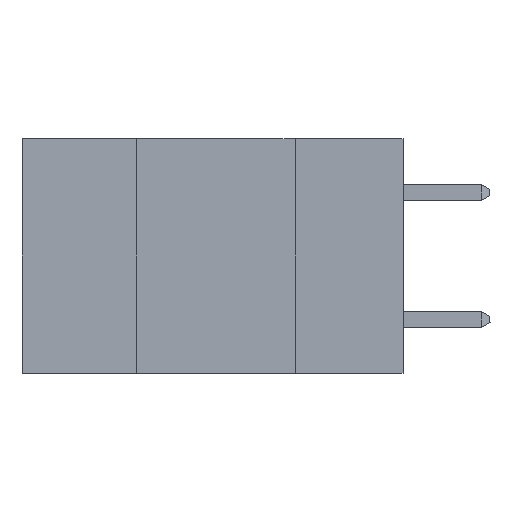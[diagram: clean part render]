
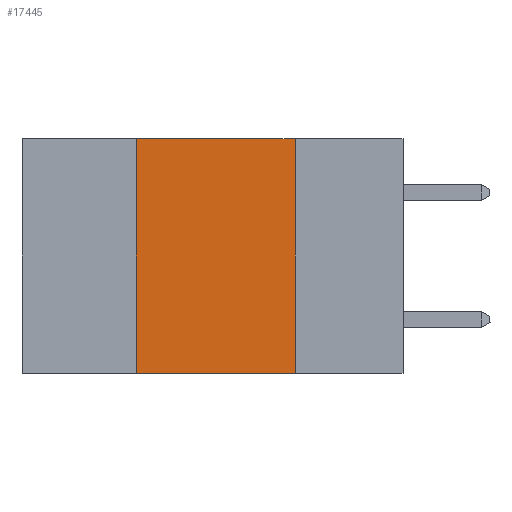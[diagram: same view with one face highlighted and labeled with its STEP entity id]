
A CAD part, left-side view. The second image highlights one B-rep face of the part: STEP entity #17445.
In plain terms, the highlighted planar face has unit normal (-1, 0, 0).
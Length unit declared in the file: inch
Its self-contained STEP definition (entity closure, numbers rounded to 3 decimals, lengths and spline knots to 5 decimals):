
#869 = EDGE_CURVE ( 'NONE', #5063, #23213, #18012, .T. ) ;
#1693 = PLANE ( 'NONE',  #20402 ) ;
#1990 = VERTEX_POINT ( 'NONE', #6628 ) ;
#2086 = CARTESIAN_POINT ( 'NONE',  ( 0., 0.17, 0. ) ) ;
#3601 = ORIENTED_EDGE ( 'NONE', *, *, #27813, .T. ) ;
#4275 = EDGE_CURVE ( 'NONE', #23213, #1990, #21564, .T. ) ;
#5063 = VERTEX_POINT ( 'NONE', #20361 ) ;
#6628 = CARTESIAN_POINT ( 'NONE',  ( 0., 0.17, 0. ) ) ;
#7242 = CARTESIAN_POINT ( 'NONE',  ( 0., 0.6, -0.37 ) ) ;
#7342 = DIRECTION ( 'NONE',  ( 0., -1., 0. ) ) ;
#7933 = EDGE_CURVE ( 'NONE', #1990, #22974, #9952, .T. ) ;
#8249 = FACE_OUTER_BOUND ( 'NONE', #17462, .T. ) ;
#9952 = LINE ( 'NONE', #2086, #22491 ) ;
#10127 = DIRECTION ( 'NONE',  ( 0., -1., 0. ) ) ;
#10980 = VECTOR ( 'NONE', #19770, 39.37008 ) ;
#11311 = CARTESIAN_POINT ( 'NONE',  ( 0., 0.6, 0. ) ) ;
#12467 = CARTESIAN_POINT ( 'NONE',  ( 0., 0.17, -0.37 ) ) ;
#16337 = ORIENTED_EDGE ( 'NONE', *, *, #869, .F. ) ;
#17445 = ADVANCED_FACE ( 'NONE', ( #8249 ), #1693, .F. ) ;
#17462 = EDGE_LOOP ( 'NONE', ( #19508, #17575, #16337, #3601 ) ) ;
#17575 = ORIENTED_EDGE ( 'NONE', *, *, #4275, .F. ) ;
#18012 = LINE ( 'NONE', #32066, #10980 ) ;
#18224 = CARTESIAN_POINT ( 'NONE',  ( 0., 0.42, 0. ) ) ;
#18865 = DIRECTION ( 'NONE',  ( 0., 0., -1. ) ) ;
#19508 = ORIENTED_EDGE ( 'NONE', *, *, #7933, .F. ) ;
#19770 = DIRECTION ( 'NONE',  ( 0., 0., 1. ) ) ;
#20361 = CARTESIAN_POINT ( 'NONE',  ( 0., 0.42, -0.37 ) ) ;
#20402 = AXIS2_PLACEMENT_3D ( 'NONE', #11311, #21623, #31371 ) ;
#21564 = LINE ( 'NONE', #25138, #29803 ) ;
#21623 = DIRECTION ( 'NONE',  ( 1., 0., 0. ) ) ;
#21707 = LINE ( 'NONE', #7242, #26742 ) ;
#22491 = VECTOR ( 'NONE', #18865, 39.37008 ) ;
#22974 = VERTEX_POINT ( 'NONE', #12467 ) ;
#23213 = VERTEX_POINT ( 'NONE', #18224 ) ;
#25138 = CARTESIAN_POINT ( 'NONE',  ( 0., 0.6, 0. ) ) ;
#26742 = VECTOR ( 'NONE', #7342, 39.37008 ) ;
#27813 = EDGE_CURVE ( 'NONE', #5063, #22974, #21707, .T. ) ;
#29803 = VECTOR ( 'NONE', #10127, 39.37008 ) ;
#31371 = DIRECTION ( 'NONE',  ( 0., 0., -1. ) ) ;
#32066 = CARTESIAN_POINT ( 'NONE',  ( 0., 0.42, 0. ) ) ;
